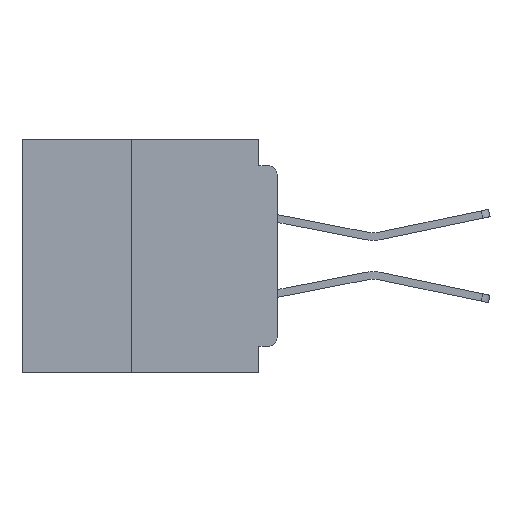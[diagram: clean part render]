
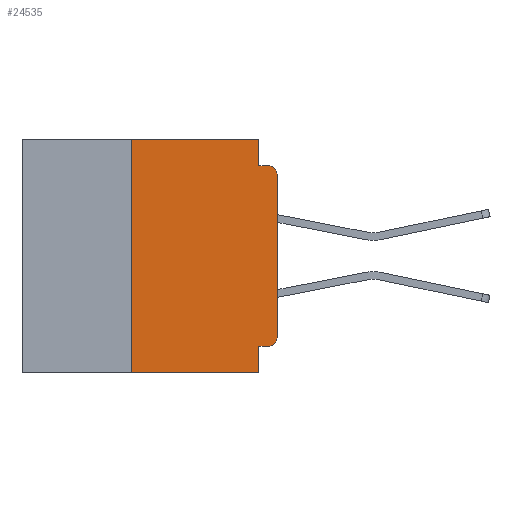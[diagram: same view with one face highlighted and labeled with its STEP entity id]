
A CAD part, left-side view. The second image highlights one B-rep face of the part: STEP entity #24535.
In plain terms, the highlighted planar face has unit normal (-1, 0, 0).
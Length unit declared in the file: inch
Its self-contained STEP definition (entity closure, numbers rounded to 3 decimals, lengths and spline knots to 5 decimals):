
#723 = CARTESIAN_POINT ( 'NONE',  ( 0., 0.015, -0.355 ) ) ;
#725 = DIRECTION ( 'NONE',  ( 0., 0., -1. ) ) ;
#1102 = AXIS2_PLACEMENT_3D ( 'NONE', #40309, #40265, #40161 ) ;
#1218 = VECTOR ( 'NONE', #29390, 39.37008 ) ;
#1500 = ORIENTED_EDGE ( 'NONE', *, *, #28502, .F. ) ;
#1542 = DIRECTION ( 'NONE',  ( 0., 0., -1. ) ) ;
#1792 = CARTESIAN_POINT ( 'NONE',  ( 0., 0., -0.045 ) ) ;
#2358 = DIRECTION ( 'NONE',  ( 0., -1., 0. ) ) ;
#3259 = DIRECTION ( 'NONE',  ( -1., 0., 0. ) ) ;
#3774 = ORIENTED_EDGE ( 'NONE', *, *, #37786, .F. ) ;
#3887 = DIRECTION ( 'NONE',  ( 0., 1., 0. ) ) ;
#4209 = LINE ( 'NONE', #7065, #11634 ) ;
#4463 = LINE ( 'NONE', #5242, #36814 ) ;
#4556 = LINE ( 'NONE', #9451, #28610 ) ;
#5242 = CARTESIAN_POINT ( 'NONE',  ( 0., 0.25, -0.4 ) ) ;
#5641 = EDGE_CURVE ( 'NONE', #12195, #8669, #26138, .T. ) ;
#5881 = VECTOR ( 'NONE', #725, 39.37008 ) ;
#6778 = CARTESIAN_POINT ( 'NONE',  ( 0., 0., -0.06 ) ) ;
#7065 = CARTESIAN_POINT ( 'NONE',  ( 0., 0., -0.355 ) ) ;
#7107 = VERTEX_POINT ( 'NONE', #22218 ) ;
#7471 = CARTESIAN_POINT ( 'NONE',  ( 0., 0.437, -0.4 ) ) ;
#7709 = CARTESIAN_POINT ( 'NONE',  ( 0., 0.015, -0.045 ) ) ;
#7766 = CARTESIAN_POINT ( 'NONE',  ( 0., 0.437, 0. ) ) ;
#8420 = CARTESIAN_POINT ( 'NONE',  ( 0., 0., -0.34 ) ) ;
#8575 = CARTESIAN_POINT ( 'NONE',  ( 0., 0.25, -0.4 ) ) ;
#8669 = VERTEX_POINT ( 'NONE', #8420 ) ;
#8976 = ORIENTED_EDGE ( 'NONE', *, *, #5641, .T. ) ;
#9451 = CARTESIAN_POINT ( 'NONE',  ( 0., 0.031, 0. ) ) ;
#9644 = LINE ( 'NONE', #7471, #1218 ) ;
#10881 = VERTEX_POINT ( 'NONE', #26388 ) ;
#11046 = EDGE_CURVE ( 'NONE', #34355, #19999, #4463, .T. ) ;
#11634 = VECTOR ( 'NONE', #3887, 39.37008 ) ;
#12195 = VERTEX_POINT ( 'NONE', #723 ) ;
#12399 = FACE_OUTER_BOUND ( 'NONE', #21598, .T. ) ;
#14564 = VERTEX_POINT ( 'NONE', #6778 ) ;
#14809 = EDGE_CURVE ( 'NONE', #33701, #36913, #30215, .T. ) ;
#14970 = CARTESIAN_POINT ( 'NONE',  ( 0., 0.031, -0.355 ) ) ;
#17641 = CARTESIAN_POINT ( 'NONE',  ( 0., 0.031, -0.045 ) ) ;
#17783 = ORIENTED_EDGE ( 'NONE', *, *, #33536, .F. ) ;
#19694 = LINE ( 'NONE', #37536, #35374 ) ;
#19999 = VERTEX_POINT ( 'NONE', #40143 ) ;
#20015 = AXIS2_PLACEMENT_3D ( 'NONE', #22073, #3259, #25218 ) ;
#20359 = DIRECTION ( 'NONE',  ( 1., 0., 0. ) ) ;
#20596 = DIRECTION ( 'NONE',  ( 0., -1., 0. ) ) ;
#21598 = EDGE_LOOP ( 'NONE', ( #25841, #24320, #38086, #3774, #39738, #23802, #31520, #17783, #1500, #8976 ) ) ;
#21869 = VECTOR ( 'NONE', #20596, 39.37008 ) ;
#22073 = CARTESIAN_POINT ( 'NONE',  ( 0., 0.015, -0.06 ) ) ;
#22218 = CARTESIAN_POINT ( 'NONE',  ( 0., 0.031, 0. ) ) ;
#22396 = CIRCLE ( 'NONE', #20015, 0.015 ) ;
#22905 = EDGE_CURVE ( 'NONE', #19999, #7107, #24267, .T. ) ;
#23802 = ORIENTED_EDGE ( 'NONE', *, *, #11046, .F. ) ;
#24148 = AXIS2_PLACEMENT_3D ( 'NONE', #7766, #20359, #1542 ) ;
#24267 = LINE ( 'NONE', #33757, #31618 ) ;
#24320 = ORIENTED_EDGE ( 'NONE', *, *, #35356, .T. ) ;
#24535 = ADVANCED_FACE ( 'NONE', ( #12399 ), #39077, .F. ) ;
#25218 = DIRECTION ( 'NONE',  ( 0., 0., -1. ) ) ;
#25841 = ORIENTED_EDGE ( 'NONE', *, *, #32759, .T. ) ;
#26138 = CIRCLE ( 'NONE', #1102, 0.015 ) ;
#26388 = CARTESIAN_POINT ( 'NONE',  ( 0., 0.031, -0.4 ) ) ;
#28502 = EDGE_CURVE ( 'NONE', #12195, #35044, #4209, .T. ) ;
#28540 = EDGE_CURVE ( 'NONE', #34355, #10881, #9644, .T. ) ;
#28610 = VECTOR ( 'NONE', #40567, 39.37008 ) ;
#29390 = DIRECTION ( 'NONE',  ( 0., -1., 0. ) ) ;
#30215 = LINE ( 'NONE', #1792, #21869 ) ;
#30892 = LINE ( 'NONE', #38307, #5881 ) ;
#31520 = ORIENTED_EDGE ( 'NONE', *, *, #28540, .T. ) ;
#31618 = VECTOR ( 'NONE', #2358, 39.37008 ) ;
#32759 = EDGE_CURVE ( 'NONE', #8669, #14564, #19694, .T. ) ;
#33480 = DIRECTION ( 'NONE',  ( 0., 0., 1. ) ) ;
#33536 = EDGE_CURVE ( 'NONE', #35044, #10881, #30892, .T. ) ;
#33701 = VERTEX_POINT ( 'NONE', #17641 ) ;
#33757 = CARTESIAN_POINT ( 'NONE',  ( 0., 0.437, 0. ) ) ;
#34355 = VERTEX_POINT ( 'NONE', #8575 ) ;
#34554 = DIRECTION ( 'NONE',  ( 0., 0., 1. ) ) ;
#35044 = VERTEX_POINT ( 'NONE', #14970 ) ;
#35356 = EDGE_CURVE ( 'NONE', #14564, #36913, #22396, .T. ) ;
#35374 = VECTOR ( 'NONE', #34554, 39.37008 ) ;
#36814 = VECTOR ( 'NONE', #33480, 39.37008 ) ;
#36913 = VERTEX_POINT ( 'NONE', #7709 ) ;
#37536 = CARTESIAN_POINT ( 'NONE',  ( 0., 0., 0. ) ) ;
#37786 = EDGE_CURVE ( 'NONE', #7107, #33701, #4556, .T. ) ;
#38086 = ORIENTED_EDGE ( 'NONE', *, *, #14809, .F. ) ;
#38307 = CARTESIAN_POINT ( 'NONE',  ( 0., 0.031, -0.4 ) ) ;
#39077 = PLANE ( 'NONE',  #24148 ) ;
#39738 = ORIENTED_EDGE ( 'NONE', *, *, #22905, .F. ) ;
#40143 = CARTESIAN_POINT ( 'NONE',  ( 0., 0.25, 0. ) ) ;
#40161 = DIRECTION ( 'NONE',  ( 0., 0., -1. ) ) ;
#40265 = DIRECTION ( 'NONE',  ( -1., 0., 0. ) ) ;
#40309 = CARTESIAN_POINT ( 'NONE',  ( 0., 0.015, -0.34 ) ) ;
#40567 = DIRECTION ( 'NONE',  ( 0., 0., -1. ) ) ;
